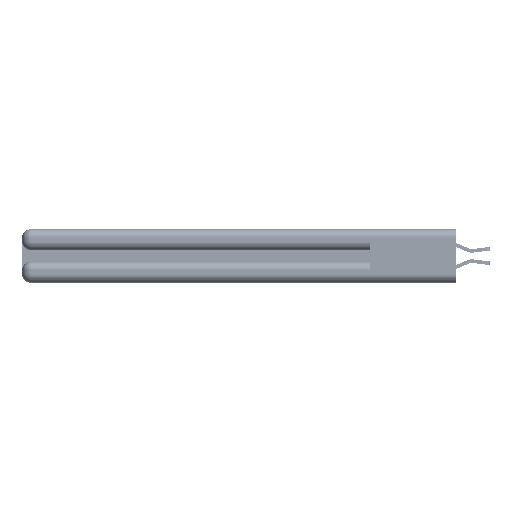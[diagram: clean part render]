
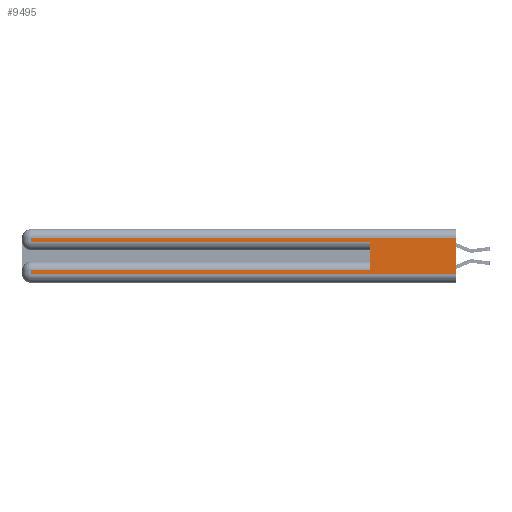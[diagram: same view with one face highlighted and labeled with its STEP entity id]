
A CAD part, left-side view. The second image highlights one B-rep face of the part: STEP entity #9495.
In plain terms, the highlighted planar face has unit normal (-1, 0, 0).
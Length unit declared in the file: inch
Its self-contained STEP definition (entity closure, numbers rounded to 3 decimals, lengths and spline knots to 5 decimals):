
#730 = EDGE_CURVE ( 'NONE', #8022, #38554, #25480, .T. ) ;
#1204 = VECTOR ( 'NONE', #49310, 39.37008 ) ;
#1824 = EDGE_CURVE ( 'NONE', #54139, #43558, #34900, .T. ) ;
#2873 = DIRECTION ( 'NONE',  ( 1., 0., 0. ) ) ;
#2876 = VERTEX_POINT ( 'NONE', #42155 ) ;
#3320 = CARTESIAN_POINT ( 'NONE',  ( 0., 0., 0.06 ) ) ;
#3398 = LINE ( 'NONE', #15824, #16542 ) ;
#3617 = VECTOR ( 'NONE', #42387, 39.37008 ) ;
#4693 = VECTOR ( 'NONE', #21953, 39.37008 ) ;
#5287 = CARTESIAN_POINT ( 'NONE',  ( 0., 2.94, 0.31 ) ) ;
#5741 = ORIENTED_EDGE ( 'NONE', *, *, #23262, .T. ) ;
#6453 = LINE ( 'NONE', #37994, #3617 ) ;
#8022 = VERTEX_POINT ( 'NONE', #5287 ) ;
#9312 = EDGE_CURVE ( 'NONE', #2876, #34792, #37605, .T. ) ;
#9495 = ADVANCED_FACE ( 'NONE', ( #28026 ), #46577, .F. ) ;
#9682 = CARTESIAN_POINT ( 'NONE',  ( 0., 0.6, 0.085 ) ) ;
#11278 = ORIENTED_EDGE ( 'NONE', *, *, #730, .T. ) ;
#12403 = CARTESIAN_POINT ( 'NONE',  ( 0., 2.94, 0.06 ) ) ;
#13364 = ORIENTED_EDGE ( 'NONE', *, *, #23611, .T. ) ;
#15824 = CARTESIAN_POINT ( 'NONE',  ( 0., 0., 0.285 ) ) ;
#16542 = VECTOR ( 'NONE', #20221, 39.37008 ) ;
#17474 = VECTOR ( 'NONE', #39552, 39.37008 ) ;
#18963 = VERTEX_POINT ( 'NONE', #39126 ) ;
#20221 = DIRECTION ( 'NONE',  ( 0., -1., 0. ) ) ;
#20878 = ORIENTED_EDGE ( 'NONE', *, *, #1824, .F. ) ;
#21953 = DIRECTION ( 'NONE',  ( 0., 0., -1. ) ) ;
#23262 = EDGE_CURVE ( 'NONE', #2876, #8022, #43475, .T. ) ;
#23611 = EDGE_CURVE ( 'NONE', #54139, #18963, #6453, .T. ) ;
#24393 = CARTESIAN_POINT ( 'NONE',  ( 0., 0., 0.06 ) ) ;
#25018 = VERTEX_POINT ( 'NONE', #12403 ) ;
#25294 = DIRECTION ( 'NONE',  ( 0., -1., 0. ) ) ;
#25463 = EDGE_CURVE ( 'NONE', #38554, #43558, #3398, .T. ) ;
#25480 = LINE ( 'NONE', #38174, #33003 ) ;
#25992 = VECTOR ( 'NONE', #54387, 39.37008 ) ;
#26623 = LINE ( 'NONE', #3320, #36873 ) ;
#27238 = EDGE_CURVE ( 'NONE', #25018, #34792, #26623, .T. ) ;
#28026 = FACE_OUTER_BOUND ( 'NONE', #41201, .T. ) ;
#29253 = CARTESIAN_POINT ( 'NONE',  ( 0., 0., 0.37 ) ) ;
#29453 = LINE ( 'NONE', #56627, #4693 ) ;
#33003 = VECTOR ( 'NONE', #42585, 39.37008 ) ;
#33398 = CARTESIAN_POINT ( 'NONE',  ( 0., 0.6, 0.285 ) ) ;
#33655 = DIRECTION ( 'NONE',  ( 0., 0., -1. ) ) ;
#34792 = VERTEX_POINT ( 'NONE', #24393 ) ;
#34900 = LINE ( 'NONE', #44957, #1204 ) ;
#35136 = AXIS2_PLACEMENT_3D ( 'NONE', #29253, #2873, #33655 ) ;
#35177 = CARTESIAN_POINT ( 'NONE',  ( 0., 0., 0.31 ) ) ;
#35210 = ORIENTED_EDGE ( 'NONE', *, *, #9312, .F. ) ;
#35995 = ORIENTED_EDGE ( 'NONE', *, *, #27238, .T. ) ;
#36873 = VECTOR ( 'NONE', #25294, 39.37008 ) ;
#37605 = LINE ( 'NONE', #49991, #25992 ) ;
#37994 = CARTESIAN_POINT ( 'NONE',  ( 0., 0., 0.085 ) ) ;
#38174 = CARTESIAN_POINT ( 'NONE',  ( 0., 2.94, 0.37 ) ) ;
#38554 = VERTEX_POINT ( 'NONE', #44107 ) ;
#38651 = ORIENTED_EDGE ( 'NONE', *, *, #25463, .T. ) ;
#39126 = CARTESIAN_POINT ( 'NONE',  ( 0., 2.94, 0.085 ) ) ;
#39552 = DIRECTION ( 'NONE',  ( 0., 1., 0. ) ) ;
#40419 = EDGE_CURVE ( 'NONE', #18963, #25018, #29453, .T. ) ;
#41201 = EDGE_LOOP ( 'NONE', ( #35210, #5741, #11278, #38651, #20878, #13364, #53658, #35995 ) ) ;
#42155 = CARTESIAN_POINT ( 'NONE',  ( 0., 0., 0.31 ) ) ;
#42387 = DIRECTION ( 'NONE',  ( 0., 1., 0. ) ) ;
#42585 = DIRECTION ( 'NONE',  ( 0., 0., -1. ) ) ;
#43475 = LINE ( 'NONE', #35177, #17474 ) ;
#43558 = VERTEX_POINT ( 'NONE', #33398 ) ;
#44107 = CARTESIAN_POINT ( 'NONE',  ( 0., 2.94, 0.285 ) ) ;
#44957 = CARTESIAN_POINT ( 'NONE',  ( 0., 0.6, 0.145 ) ) ;
#46577 = PLANE ( 'NONE',  #35136 ) ;
#49310 = DIRECTION ( 'NONE',  ( 0., 0., 1. ) ) ;
#49991 = CARTESIAN_POINT ( 'NONE',  ( 0., 0., 0.37 ) ) ;
#53658 = ORIENTED_EDGE ( 'NONE', *, *, #40419, .T. ) ;
#54139 = VERTEX_POINT ( 'NONE', #9682 ) ;
#54387 = DIRECTION ( 'NONE',  ( 0., 0., -1. ) ) ;
#56627 = CARTESIAN_POINT ( 'NONE',  ( 0., 2.94, 0.37 ) ) ;
